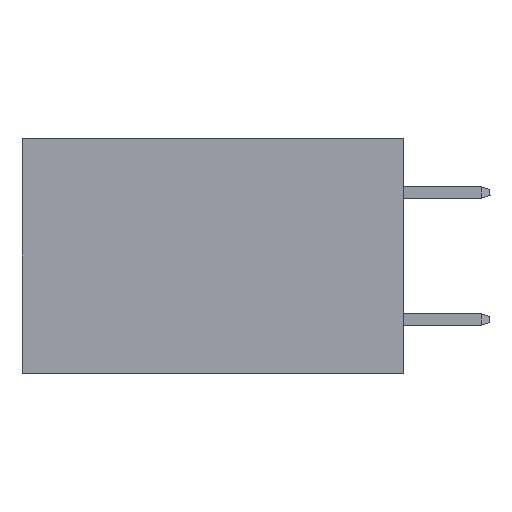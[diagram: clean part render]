
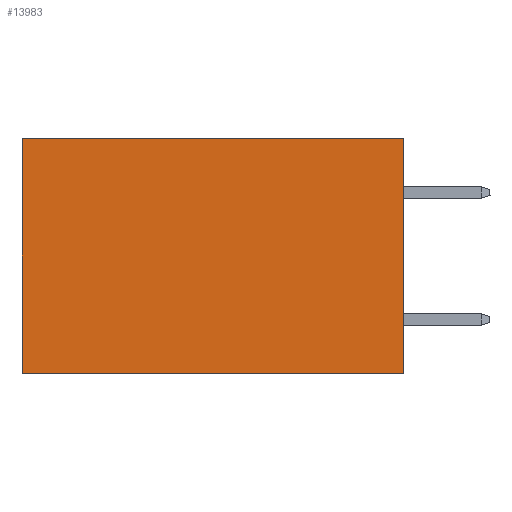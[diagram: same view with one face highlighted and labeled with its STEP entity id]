
A CAD part, left-side view. The second image highlights one B-rep face of the part: STEP entity #13983.
In plain terms, the highlighted planar face has unit normal (-1, 0, 0).
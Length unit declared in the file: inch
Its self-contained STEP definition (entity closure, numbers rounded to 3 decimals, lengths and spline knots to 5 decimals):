
#1344 = EDGE_CURVE ( 'NONE', #3945, #15107, #27320, .T. ) ;
#1396 = EDGE_CURVE ( 'NONE', #15107, #22756, #4858, .T. ) ;
#1610 = LINE ( 'NONE', #33195, #7024 ) ;
#2529 = CARTESIAN_POINT ( 'NONE',  ( 0.2875, 0.6, 0. ) ) ;
#2698 = CARTESIAN_POINT ( 'NONE',  ( 0.2875, 0., 0. ) ) ;
#3945 = VERTEX_POINT ( 'NONE', #2698 ) ;
#4108 = EDGE_CURVE ( 'NONE', #3945, #12070, #4748, .T. ) ;
#4748 = LINE ( 'NONE', #22510, #25557 ) ;
#4858 = LINE ( 'NONE', #30587, #16595 ) ;
#5829 = FACE_OUTER_BOUND ( 'NONE', #23988, .T. ) ;
#6348 = DIRECTION ( 'NONE',  ( 0., 0., -1. ) ) ;
#6410 = EDGE_CURVE ( 'NONE', #12070, #22756, #1610, .T. ) ;
#6993 = DIRECTION ( 'NONE',  ( 0., 1., 0. ) ) ;
#7024 = VECTOR ( 'NONE', #20055, 39.37008 ) ;
#9361 = DIRECTION ( 'NONE',  ( 0., 0., -1. ) ) ;
#12070 = VERTEX_POINT ( 'NONE', #2529 ) ;
#13582 = PLANE ( 'NONE',  #32325 ) ;
#13983 = ADVANCED_FACE ( 'NONE', ( #5829 ), #13582, .F. ) ;
#15107 = VERTEX_POINT ( 'NONE', #23798 ) ;
#16345 = CARTESIAN_POINT ( 'NONE',  ( 0.2875, 0., 0. ) ) ;
#16595 = VECTOR ( 'NONE', #33177, 39.37008 ) ;
#18679 = VECTOR ( 'NONE', #9361, 39.37008 ) ;
#20055 = DIRECTION ( 'NONE',  ( 0., 0., -1. ) ) ;
#22510 = CARTESIAN_POINT ( 'NONE',  ( 0.2875, 0., 0. ) ) ;
#22756 = VERTEX_POINT ( 'NONE', #25761 ) ;
#23798 = CARTESIAN_POINT ( 'NONE',  ( 0.2875, 0., -0.37 ) ) ;
#23988 = EDGE_LOOP ( 'NONE', ( #24585, #24100, #26072, #33129 ) ) ;
#24100 = ORIENTED_EDGE ( 'NONE', *, *, #1396, .F. ) ;
#24585 = ORIENTED_EDGE ( 'NONE', *, *, #6410, .T. ) ;
#25557 = VECTOR ( 'NONE', #6993, 39.37008 ) ;
#25761 = CARTESIAN_POINT ( 'NONE',  ( 0.2875, 0.6, -0.37 ) ) ;
#26072 = ORIENTED_EDGE ( 'NONE', *, *, #1344, .F. ) ;
#27141 = CARTESIAN_POINT ( 'NONE',  ( 0.2875, 0., 0. ) ) ;
#27320 = LINE ( 'NONE', #27141, #18679 ) ;
#30587 = CARTESIAN_POINT ( 'NONE',  ( 0.2875, 0., -0.37 ) ) ;
#32242 = DIRECTION ( 'NONE',  ( 1., 0., 0. ) ) ;
#32325 = AXIS2_PLACEMENT_3D ( 'NONE', #16345, #32242, #6348 ) ;
#33129 = ORIENTED_EDGE ( 'NONE', *, *, #4108, .T. ) ;
#33177 = DIRECTION ( 'NONE',  ( 0., 1., 0. ) ) ;
#33195 = CARTESIAN_POINT ( 'NONE',  ( 0.2875, 0.6, 0. ) ) ;
